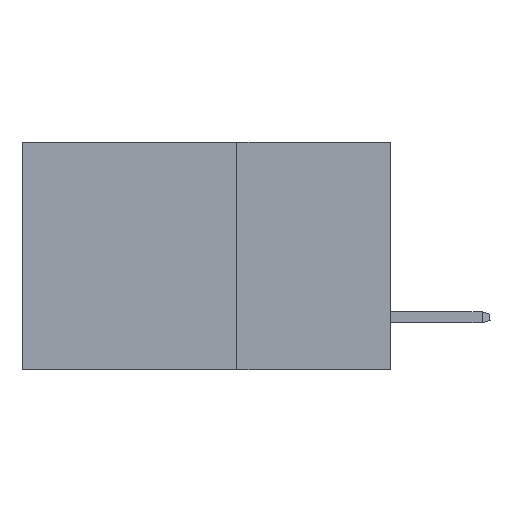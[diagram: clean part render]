
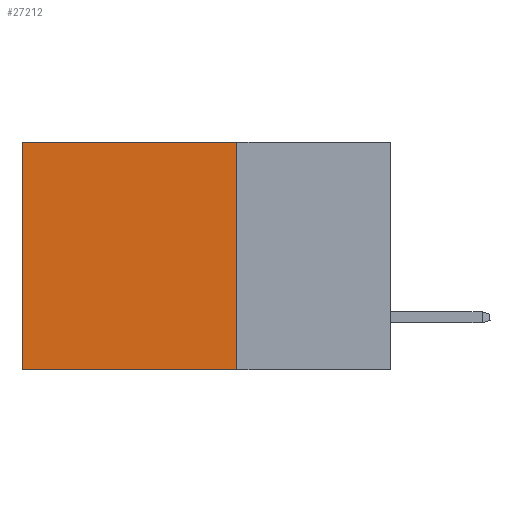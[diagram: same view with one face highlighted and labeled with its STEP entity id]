
A CAD part, left-side view. The second image highlights one B-rep face of the part: STEP entity #27212.
In plain terms, the highlighted planar face has unit normal (-1, 0, 0).
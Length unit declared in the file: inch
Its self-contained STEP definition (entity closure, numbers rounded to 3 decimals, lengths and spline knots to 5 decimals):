
#896 = LINE ( 'NONE', #22415, #40717 ) ;
#918 = EDGE_LOOP ( 'NONE', ( #37324, #10307, #6970, #11450 ) ) ;
#4449 = DIRECTION ( 'NONE',  ( 0., 1., 0. ) ) ;
#4621 = VERTEX_POINT ( 'NONE', #29737 ) ;
#4735 = EDGE_CURVE ( 'NONE', #19143, #43103, #4805, .T. ) ;
#4805 = LINE ( 'NONE', #23631, #19579 ) ;
#5834 = DIRECTION ( 'NONE',  ( 0., 1., 0. ) ) ;
#6970 = ORIENTED_EDGE ( 'NONE', *, *, #4735, .F. ) ;
#7160 = VECTOR ( 'NONE', #4449, 39.37008 ) ;
#9092 = PLANE ( 'NONE',  #12478 ) ;
#10307 = ORIENTED_EDGE ( 'NONE', *, *, #41688, .F. ) ;
#11450 = ORIENTED_EDGE ( 'NONE', *, *, #24682, .T. ) ;
#12478 = AXIS2_PLACEMENT_3D ( 'NONE', #32880, #27448, #42109 ) ;
#19143 = VERTEX_POINT ( 'NONE', #40716 ) ;
#19526 = EDGE_CURVE ( 'NONE', #4621, #30006, #32614, .T. ) ;
#19579 = VECTOR ( 'NONE', #23333, 39.37008 ) ;
#22415 = CARTESIAN_POINT ( 'NONE',  ( 0.2875, 0.25, 0. ) ) ;
#23333 = DIRECTION ( 'NONE',  ( 0., 0., -1. ) ) ;
#23631 = CARTESIAN_POINT ( 'NONE',  ( 0.2875, 0.25, 0. ) ) ;
#24682 = EDGE_CURVE ( 'NONE', #19143, #4621, #896, .T. ) ;
#24738 = CARTESIAN_POINT ( 'NONE',  ( 0.2875, 0.25, -0.37 ) ) ;
#25227 = LINE ( 'NONE', #24738, #7160 ) ;
#27212 = ADVANCED_FACE ( 'NONE', ( #36150 ), #9092, .F. ) ;
#27448 = DIRECTION ( 'NONE',  ( 1., 0., 0. ) ) ;
#29737 = CARTESIAN_POINT ( 'NONE',  ( 0.2875, 0.6, 0. ) ) ;
#30006 = VERTEX_POINT ( 'NONE', #30056 ) ;
#30056 = CARTESIAN_POINT ( 'NONE',  ( 0.2875, 0.6, -0.37 ) ) ;
#32614 = LINE ( 'NONE', #38625, #40590 ) ;
#32880 = CARTESIAN_POINT ( 'NONE',  ( 0.2875, 0.25, 0. ) ) ;
#36150 = FACE_OUTER_BOUND ( 'NONE', #918, .T. ) ;
#37324 = ORIENTED_EDGE ( 'NONE', *, *, #19526, .T. ) ;
#38625 = CARTESIAN_POINT ( 'NONE',  ( 0.2875, 0.6, 0. ) ) ;
#39642 = DIRECTION ( 'NONE',  ( 0., 0., -1. ) ) ;
#40590 = VECTOR ( 'NONE', #39642, 39.37008 ) ;
#40716 = CARTESIAN_POINT ( 'NONE',  ( 0.2875, 0.25, 0. ) ) ;
#40717 = VECTOR ( 'NONE', #5834, 39.37008 ) ;
#41067 = CARTESIAN_POINT ( 'NONE',  ( 0.2875, 0.25, -0.37 ) ) ;
#41688 = EDGE_CURVE ( 'NONE', #43103, #30006, #25227, .T. ) ;
#42109 = DIRECTION ( 'NONE',  ( 0., 0., -1. ) ) ;
#43103 = VERTEX_POINT ( 'NONE', #41067 ) ;
